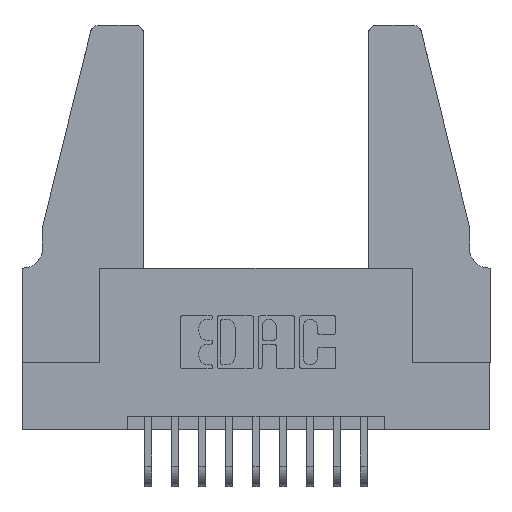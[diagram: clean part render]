
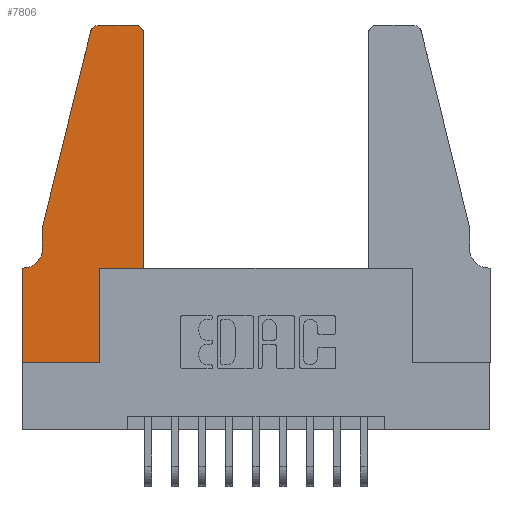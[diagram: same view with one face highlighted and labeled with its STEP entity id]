
A CAD part, top view. The second image highlights one B-rep face of the part: STEP entity #7806.
In plain terms, the highlighted planar face has unit normal (0, 0, 1).
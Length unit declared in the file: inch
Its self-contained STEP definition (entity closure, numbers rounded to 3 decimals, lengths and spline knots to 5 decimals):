
#333 = VERTEX_POINT ( 'NONE', #9240 ) ;
#415 = DIRECTION ( 'NONE',  ( 0., 0., 1. ) ) ;
#424 = VECTOR ( 'NONE', #2463, 39.37008 ) ;
#523 = VERTEX_POINT ( 'NONE', #8155 ) ;
#778 = CARTESIAN_POINT ( 'NONE',  ( 0.284, 1.22, 0.37 ) ) ;
#1206 = CARTESIAN_POINT ( 'NONE',  ( 0., 0., 0.37 ) ) ;
#1234 = ORIENTED_EDGE ( 'NONE', *, *, #8428, .T. ) ;
#1591 = VECTOR ( 'NONE', #5999, 39.37008 ) ;
#1643 = DIRECTION ( 'NONE',  ( 1., 0., 0. ) ) ;
#1732 = DIRECTION ( 'NONE',  ( 0., 0., -1. ) ) ;
#1749 = VERTEX_POINT ( 'NONE', #6968 ) ;
#2403 = CARTESIAN_POINT ( 'NONE',  ( 0.0055, 0.35, 0.37 ) ) ;
#2463 = DIRECTION ( 'NONE',  ( 0., 1., 0. ) ) ;
#2539 = EDGE_CURVE ( 'NONE', #10841, #15034, #6461, .T. ) ;
#2650 = ORIENTED_EDGE ( 'NONE', *, *, #3404, .T. ) ;
#2736 = VECTOR ( 'NONE', #5961, 39.37008 ) ;
#2994 = AXIS2_PLACEMENT_3D ( 'NONE', #4108, #1732, #7642 ) ;
#3390 = CARTESIAN_POINT ( 'NONE',  ( 0.0755, 0.42, 0.37 ) ) ;
#3404 = EDGE_CURVE ( 'NONE', #523, #15286, #7948, .T. ) ;
#3429 = CARTESIAN_POINT ( 'NONE',  ( 0.25487, 1.22718, 0.37 ) ) ;
#3465 = ORIENTED_EDGE ( 'NONE', *, *, #6567, .T. ) ;
#3532 = CARTESIAN_POINT ( 'NONE',  ( 0.4505, 0.35, 0.37 ) ) ;
#3554 = CARTESIAN_POINT ( 'NONE',  ( 0.4505, 1.22, 0.37 ) ) ;
#3706 = CARTESIAN_POINT ( 'NONE',  ( 0.4505, 0.35, 0.37 ) ) ;
#3881 = CARTESIAN_POINT ( 'NONE',  ( 0.2865, 0.35, 0.37 ) ) ;
#4048 = CARTESIAN_POINT ( 'NONE',  ( 0.4505, 0.35, 0.37 ) ) ;
#4106 = ORIENTED_EDGE ( 'NONE', *, *, #2539, .T. ) ;
#4108 = CARTESIAN_POINT ( 'NONE',  ( 0.0055, 0.42, 0.37 ) ) ;
#4171 = EDGE_CURVE ( 'NONE', #15286, #7078, #7349, .T. ) ;
#4201 = VECTOR ( 'NONE', #5164, 39.37008 ) ;
#4212 = ORIENTED_EDGE ( 'NONE', *, *, #9658, .T. ) ;
#4409 = AXIS2_PLACEMENT_3D ( 'NONE', #778, #15025, #11361 ) ;
#4415 = VECTOR ( 'NONE', #5327, 39.37008 ) ;
#4646 = CIRCLE ( 'NONE', #4409, 0.03 ) ;
#5035 = ORIENTED_EDGE ( 'NONE', *, *, #15174, .T. ) ;
#5137 = LINE ( 'NONE', #12366, #4415 ) ;
#5164 = DIRECTION ( 'NONE',  ( 0., 1., 0. ) ) ;
#5209 = LINE ( 'NONE', #3706, #424 ) ;
#5327 = DIRECTION ( 'NONE',  ( 0., -1., 0. ) ) ;
#5674 = FACE_OUTER_BOUND ( 'NONE', #10855, .T. ) ;
#5961 = DIRECTION ( 'NONE',  ( 1., 0., 0. ) ) ;
#5999 = DIRECTION ( 'NONE',  ( 1., 0., 0. ) ) ;
#6461 = CIRCLE ( 'NONE', #15178, 0.03 ) ;
#6567 = EDGE_CURVE ( 'NONE', #333, #523, #5137, .T. ) ;
#6742 = CARTESIAN_POINT ( 'NONE',  ( 0.2865, 0.35, 0.37 ) ) ;
#6921 = VERTEX_POINT ( 'NONE', #3390 ) ;
#6968 = CARTESIAN_POINT ( 'NONE',  ( 0.0755, 0.5, 0.37 ) ) ;
#7078 = VERTEX_POINT ( 'NONE', #6742 ) ;
#7094 = CARTESIAN_POINT ( 'NONE',  ( 0.0755, 0.5, 0.37 ) ) ;
#7154 = AXIS2_PLACEMENT_3D ( 'NONE', #7495, #415, #1643 ) ;
#7195 = CARTESIAN_POINT ( 'NONE',  ( 0.4205, 1.25, 0.37 ) ) ;
#7304 = LINE ( 'NONE', #14492, #15289 ) ;
#7327 = LINE ( 'NONE', #7094, #14555 ) ;
#7349 = LINE ( 'NONE', #3881, #4201 ) ;
#7495 = CARTESIAN_POINT ( 'NONE',  ( 0., 0.35, 0.37 ) ) ;
#7642 = DIRECTION ( 'NONE',  ( -1., 0., 0. ) ) ;
#7696 = ORIENTED_EDGE ( 'NONE', *, *, #4171, .T. ) ;
#7740 = ORIENTED_EDGE ( 'NONE', *, *, #13362, .T. ) ;
#7806 = ADVANCED_FACE ( 'NONE', ( #5674 ), #14598, .T. ) ;
#7826 = CARTESIAN_POINT ( 'NONE',  ( 0.2865, 0., 0.37 ) ) ;
#7896 = ORIENTED_EDGE ( 'NONE', *, *, #11465, .T. ) ;
#7910 = LINE ( 'NONE', #3532, #1591 ) ;
#7948 = LINE ( 'NONE', #1206, #2736 ) ;
#8133 = EDGE_CURVE ( 'NONE', #7078, #12268, #7910, .T. ) ;
#8155 = CARTESIAN_POINT ( 'NONE',  ( 0., 0., 0.37 ) ) ;
#8254 = VERTEX_POINT ( 'NONE', #2403 ) ;
#8428 = EDGE_CURVE ( 'NONE', #1749, #6921, #7327, .T. ) ;
#8541 = DIRECTION ( 'NONE',  ( 0., 0., 1. ) ) ;
#8586 = ORIENTED_EDGE ( 'NONE', *, *, #11204, .T. ) ;
#8695 = ORIENTED_EDGE ( 'NONE', *, *, #8133, .T. ) ;
#8816 = VERTEX_POINT ( 'NONE', #3429 ) ;
#9027 = EDGE_CURVE ( 'NONE', #8816, #1749, #13614, .T. ) ;
#9240 = CARTESIAN_POINT ( 'NONE',  ( 0., 0.35, 0.37 ) ) ;
#9658 = EDGE_CURVE ( 'NONE', #6921, #8254, #12073, .T. ) ;
#9755 = DIRECTION ( 'NONE',  ( 1., 0., 0. ) ) ;
#9892 = CARTESIAN_POINT ( 'NONE',  ( 0.0755, 0.35, 0.37 ) ) ;
#10761 = LINE ( 'NONE', #9892, #11682 ) ;
#10841 = VERTEX_POINT ( 'NONE', #3554 ) ;
#10855 = EDGE_LOOP ( 'NONE', ( #7740, #7896, #11500, #1234, #4212, #5035, #3465, #2650, #7696, #8695, #8586, #4106 ) ) ;
#10959 = CARTESIAN_POINT ( 'NONE',  ( 0.4205, 1.22, 0.37 ) ) ;
#11204 = EDGE_CURVE ( 'NONE', #12268, #10841, #5209, .T. ) ;
#11338 = VERTEX_POINT ( 'NONE', #12050 ) ;
#11361 = DIRECTION ( 'NONE',  ( 1., 0., 0. ) ) ;
#11465 = EDGE_CURVE ( 'NONE', #11338, #8816, #4646, .T. ) ;
#11500 = ORIENTED_EDGE ( 'NONE', *, *, #9027, .T. ) ;
#11682 = VECTOR ( 'NONE', #12145, 39.37008 ) ;
#11737 = CARTESIAN_POINT ( 'NONE',  ( 0.0755, 0.5, 0.37 ) ) ;
#11792 = DIRECTION ( 'NONE',  ( 0., -1., 0. ) ) ;
#12050 = CARTESIAN_POINT ( 'NONE',  ( 0.284, 1.25, 0.37 ) ) ;
#12073 = CIRCLE ( 'NONE', #2994, 0.07 ) ;
#12145 = DIRECTION ( 'NONE',  ( -1., 0., 0. ) ) ;
#12196 = DIRECTION ( 'NONE',  ( -1., 0., 0. ) ) ;
#12268 = VERTEX_POINT ( 'NONE', #4048 ) ;
#12366 = CARTESIAN_POINT ( 'NONE',  ( 0., 0., 0.37 ) ) ;
#13362 = EDGE_CURVE ( 'NONE', #15034, #11338, #7304, .T. ) ;
#13614 = LINE ( 'NONE', #11737, #13795 ) ;
#13795 = VECTOR ( 'NONE', #14189, 39.37008 ) ;
#14189 = DIRECTION ( 'NONE',  ( -0.239, -0.971, 0. ) ) ;
#14492 = CARTESIAN_POINT ( 'NONE',  ( 0.2605, 1.25, 0.37 ) ) ;
#14555 = VECTOR ( 'NONE', #11792, 39.37008 ) ;
#14598 = PLANE ( 'NONE',  #7154 ) ;
#15025 = DIRECTION ( 'NONE',  ( 0., 0., 1. ) ) ;
#15034 = VERTEX_POINT ( 'NONE', #7195 ) ;
#15174 = EDGE_CURVE ( 'NONE', #8254, #333, #10761, .T. ) ;
#15178 = AXIS2_PLACEMENT_3D ( 'NONE', #10959, #8541, #9755 ) ;
#15286 = VERTEX_POINT ( 'NONE', #7826 ) ;
#15289 = VECTOR ( 'NONE', #12196, 39.37008 ) ;
